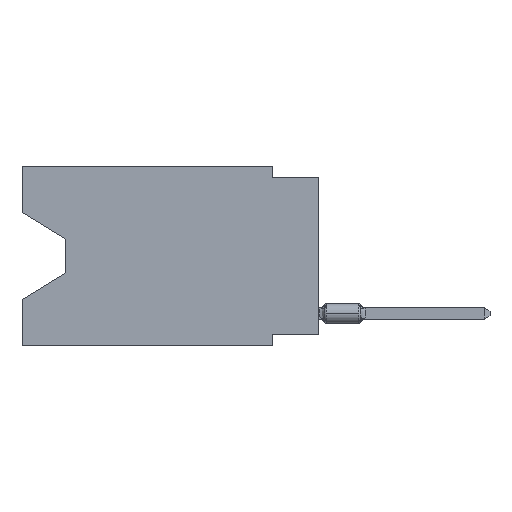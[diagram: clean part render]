
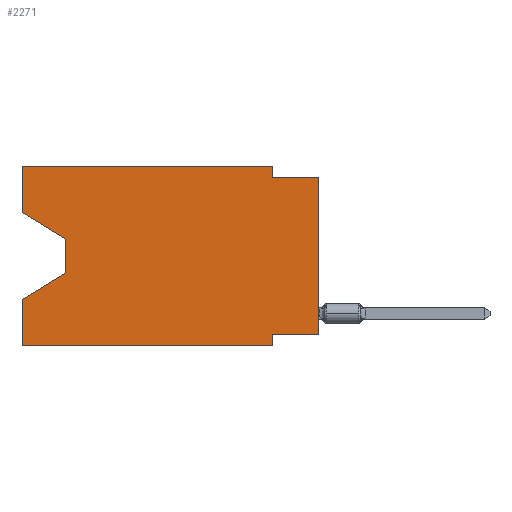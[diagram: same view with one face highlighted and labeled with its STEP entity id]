
A CAD part, left-side view. The second image highlights one B-rep face of the part: STEP entity #2271.
In plain terms, the highlighted planar face has unit normal (-1, 0, 0).
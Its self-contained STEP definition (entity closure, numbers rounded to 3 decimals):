
#328 = VECTOR ( 'NONE', #9756, 1000. ) ;
#587 = DIRECTION ( 'NONE',  ( 0., 1., 0. ) ) ;
#646 = AXIS2_PLACEMENT_3D ( 'NONE', #6576, #3725, #17862 ) ;
#699 = CARTESIAN_POINT ( 'NONE',  ( 0., 16.383, 0. ) ) ;
#760 = VECTOR ( 'NONE', #2151, 1000. ) ;
#955 = VERTEX_POINT ( 'NONE', #3458 ) ;
#1020 = EDGE_CURVE ( 'NONE', #9786, #955, #10926, .T. ) ;
#1961 = VECTOR ( 'NONE', #4244, 1000. ) ;
#1993 = LINE ( 'NONE', #7620, #8667 ) ;
#2128 = EDGE_CURVE ( 'NONE', #12968, #10852, #9191, .T. ) ;
#2151 = DIRECTION ( 'NONE',  ( 0., -1., 0. ) ) ;
#2271 = ADVANCED_FACE ( 'NONE', ( #13990 ), #5556, .F. ) ;
#2492 = VECTOR ( 'NONE', #5087, 1000. ) ;
#2599 = VERTEX_POINT ( 'NONE', #17104 ) ;
#2794 = CARTESIAN_POINT ( 'NONE',  ( 0., 16.383, -2.546 ) ) ;
#2991 = ORIENTED_EDGE ( 'NONE', *, *, #7209, .T. ) ;
#3047 = DIRECTION ( 'NONE',  ( 0., 0., -1. ) ) ;
#3061 = ORIENTED_EDGE ( 'NONE', *, *, #3518, .F. ) ;
#3107 = VECTOR ( 'NONE', #11758, 1000. ) ;
#3447 = ORIENTED_EDGE ( 'NONE', *, *, #15939, .F. ) ;
#3458 = CARTESIAN_POINT ( 'NONE',  ( 0., 2.54, 0. ) ) ;
#3518 = EDGE_CURVE ( 'NONE', #12968, #8736, #1993, .T. ) ;
#3721 = CARTESIAN_POINT ( 'NONE',  ( 0., 16.383, 0. ) ) ;
#3725 = DIRECTION ( 'NONE',  ( 1., 0., 0. ) ) ;
#3906 = VECTOR ( 'NONE', #3047, 1000. ) ;
#3934 = CARTESIAN_POINT ( 'NONE',  ( 0., 0., -9.271 ) ) ;
#4097 = LINE ( 'NONE', #2794, #328 ) ;
#4244 = DIRECTION ( 'NONE',  ( 0., 0.855, -0.519 ) ) ;
#4324 = CARTESIAN_POINT ( 'NONE',  ( 0., 13.97, -4.013 ) ) ;
#4816 = EDGE_CURVE ( 'NONE', #7741, #14965, #4097, .T. ) ;
#4913 = CARTESIAN_POINT ( 'NONE',  ( 0., 0., -0.635 ) ) ;
#5087 = DIRECTION ( 'NONE',  ( 0., -1., 0. ) ) ;
#5221 = VECTOR ( 'NONE', #16338, 1000. ) ;
#5370 = EDGE_CURVE ( 'NONE', #12011, #12460, #16917, .T. ) ;
#5556 = PLANE ( 'NONE',  #646 ) ;
#5714 = VECTOR ( 'NONE', #12848, 1000. ) ;
#6108 = LINE ( 'NONE', #12957, #3906 ) ;
#6158 = ORIENTED_EDGE ( 'NONE', *, *, #4816, .T. ) ;
#6576 = CARTESIAN_POINT ( 'NONE',  ( 0., 16.383, 0. ) ) ;
#7209 = EDGE_CURVE ( 'NONE', #14965, #12011, #11881, .T. ) ;
#7306 = ORIENTED_EDGE ( 'NONE', *, *, #5370, .T. ) ;
#7552 = VECTOR ( 'NONE', #15454, 1000. ) ;
#7606 = EDGE_CURVE ( 'NONE', #2599, #13442, #8819, .T. ) ;
#7620 = CARTESIAN_POINT ( 'NONE',  ( 0., 0., -9.271 ) ) ;
#7626 = CARTESIAN_POINT ( 'NONE',  ( 0., 13.97, -5.893 ) ) ;
#7741 = VERTEX_POINT ( 'NONE', #15025 ) ;
#7771 = EDGE_CURVE ( 'NONE', #955, #11177, #10089, .T. ) ;
#7885 = ORIENTED_EDGE ( 'NONE', *, *, #11726, .F. ) ;
#8667 = VECTOR ( 'NONE', #587, 1000. ) ;
#8694 = CARTESIAN_POINT ( 'NONE',  ( 0., 13.97, -5.893 ) ) ;
#8736 = VERTEX_POINT ( 'NONE', #14390 ) ;
#8819 = LINE ( 'NONE', #12052, #760 ) ;
#8902 = DIRECTION ( 'NONE',  ( 0., 0., 1. ) ) ;
#9079 = LINE ( 'NONE', #11924, #3107 ) ;
#9191 = LINE ( 'NONE', #17417, #16990 ) ;
#9756 = DIRECTION ( 'NONE',  ( 0., -0.855, -0.519 ) ) ;
#9786 = VERTEX_POINT ( 'NONE', #13581 ) ;
#10089 = LINE ( 'NONE', #12959, #7552 ) ;
#10142 = ORIENTED_EDGE ( 'NONE', *, *, #7606, .T. ) ;
#10325 = CARTESIAN_POINT ( 'NONE',  ( 0., 13.97, -4.013 ) ) ;
#10587 = ORIENTED_EDGE ( 'NONE', *, *, #1020, .F. ) ;
#10852 = VERTEX_POINT ( 'NONE', #4913 ) ;
#10926 = LINE ( 'NONE', #3721, #2492 ) ;
#11177 = VERTEX_POINT ( 'NONE', #17562 ) ;
#11465 = LINE ( 'NONE', #15726, #5714 ) ;
#11490 = ORIENTED_EDGE ( 'NONE', *, *, #7771, .F. ) ;
#11726 = EDGE_CURVE ( 'NONE', #2599, #12460, #16604, .T. ) ;
#11758 = DIRECTION ( 'NONE',  ( 0., 0., 1. ) ) ;
#11881 = LINE ( 'NONE', #10325, #11979 ) ;
#11924 = CARTESIAN_POINT ( 'NONE',  ( 0., 16.383, 0. ) ) ;
#11979 = VECTOR ( 'NONE', #17707, 1000. ) ;
#11998 = ORIENTED_EDGE ( 'NONE', *, *, #17391, .F. ) ;
#12011 = VERTEX_POINT ( 'NONE', #7626 ) ;
#12052 = CARTESIAN_POINT ( 'NONE',  ( 0., 16.383, -9.906 ) ) ;
#12407 = EDGE_CURVE ( 'NONE', #7741, #9786, #9079, .T. ) ;
#12460 = VERTEX_POINT ( 'NONE', #13042 ) ;
#12848 = DIRECTION ( 'NONE',  ( 0., -1., 0. ) ) ;
#12957 = CARTESIAN_POINT ( 'NONE',  ( 0., 2.54, -9.906 ) ) ;
#12959 = CARTESIAN_POINT ( 'NONE',  ( 0., 2.54, 0. ) ) ;
#12968 = VERTEX_POINT ( 'NONE', #3934 ) ;
#13042 = CARTESIAN_POINT ( 'NONE',  ( 0., 16.383, -7.36 ) ) ;
#13442 = VERTEX_POINT ( 'NONE', #16244 ) ;
#13581 = CARTESIAN_POINT ( 'NONE',  ( 0., 16.383, 0. ) ) ;
#13990 = FACE_OUTER_BOUND ( 'NONE', #14967, .T. ) ;
#14390 = CARTESIAN_POINT ( 'NONE',  ( 0., 2.54, -9.271 ) ) ;
#14965 = VERTEX_POINT ( 'NONE', #4324 ) ;
#14967 = EDGE_LOOP ( 'NONE', ( #6158, #2991, #7306, #7885, #10142, #3447, #3061, #15692, #11998, #11490, #10587, #17098 ) ) ;
#15025 = CARTESIAN_POINT ( 'NONE',  ( 0., 16.383, -2.546 ) ) ;
#15454 = DIRECTION ( 'NONE',  ( 0., 0., -1. ) ) ;
#15692 = ORIENTED_EDGE ( 'NONE', *, *, #2128, .T. ) ;
#15726 = CARTESIAN_POINT ( 'NONE',  ( 0., 0., -0.635 ) ) ;
#15939 = EDGE_CURVE ( 'NONE', #8736, #13442, #6108, .T. ) ;
#16244 = CARTESIAN_POINT ( 'NONE',  ( 0., 2.54, -9.906 ) ) ;
#16338 = DIRECTION ( 'NONE',  ( 0., 0., 1. ) ) ;
#16604 = LINE ( 'NONE', #699, #5221 ) ;
#16917 = LINE ( 'NONE', #8694, #1961 ) ;
#16990 = VECTOR ( 'NONE', #8902, 1000. ) ;
#17098 = ORIENTED_EDGE ( 'NONE', *, *, #12407, .F. ) ;
#17104 = CARTESIAN_POINT ( 'NONE',  ( 0., 16.383, -9.906 ) ) ;
#17391 = EDGE_CURVE ( 'NONE', #11177, #10852, #11465, .T. ) ;
#17417 = CARTESIAN_POINT ( 'NONE',  ( 0., 0., 0. ) ) ;
#17562 = CARTESIAN_POINT ( 'NONE',  ( 0., 2.54, -0.635 ) ) ;
#17707 = DIRECTION ( 'NONE',  ( 0., 0., -1. ) ) ;
#17862 = DIRECTION ( 'NONE',  ( 0., 0., -1. ) ) ;
